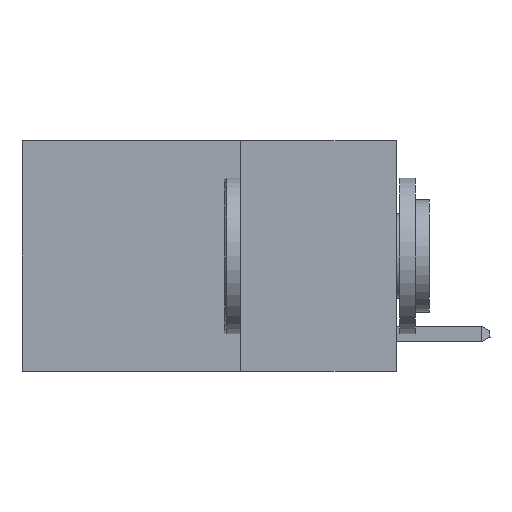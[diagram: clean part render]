
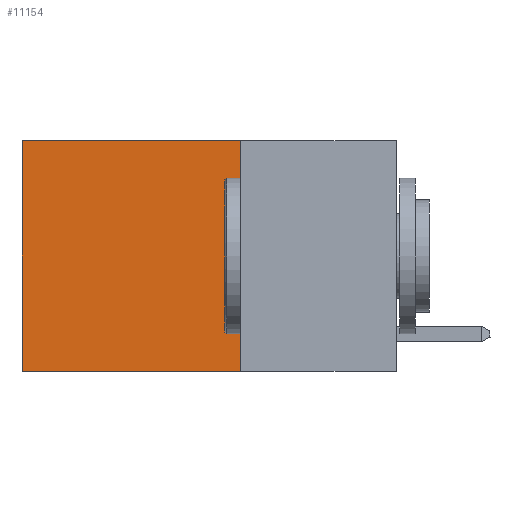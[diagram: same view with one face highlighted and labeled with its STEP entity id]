
A CAD part, left-side view. The second image highlights one B-rep face of the part: STEP entity #11154.
In plain terms, the highlighted planar face has unit normal (-1, 0, 0).
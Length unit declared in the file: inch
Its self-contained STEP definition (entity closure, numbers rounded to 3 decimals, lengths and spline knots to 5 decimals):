
#129 = ORIENTED_EDGE ( 'NONE', *, *, #913, .T. ) ;
#226 = ORIENTED_EDGE ( 'NONE', *, *, #10465, .F. ) ;
#417 = ORIENTED_EDGE ( 'NONE', *, *, #9781, .F. ) ;
#844 = ORIENTED_EDGE ( 'NONE', *, *, #8347, .T. ) ;
#913 = EDGE_CURVE ( 'NONE', #7312, #3012, #1045, .T. ) ;
#1045 = LINE ( 'NONE', #1157, #8351 ) ;
#1157 = CARTESIAN_POINT ( 'NONE',  ( 0.2625, 0.6, 0. ) ) ;
#1704 = DIRECTION ( 'NONE',  ( 1., 0., 0. ) ) ;
#1806 = DIRECTION ( 'NONE',  ( 0., 1., 0. ) ) ;
#2155 = VERTEX_POINT ( 'NONE', #4856 ) ;
#2411 = CARTESIAN_POINT ( 'NONE',  ( 0.2625, 0.6, 0. ) ) ;
#2602 = CARTESIAN_POINT ( 'NONE',  ( 0.2625, 0.25, 0. ) ) ;
#2667 = CARTESIAN_POINT ( 'NONE',  ( 0.2625, 0.25, -0.37 ) ) ;
#3012 = VERTEX_POINT ( 'NONE', #6896 ) ;
#3633 = VERTEX_POINT ( 'NONE', #2667 ) ;
#4054 = CARTESIAN_POINT ( 'NONE',  ( 0.2625, 0.25, 0. ) ) ;
#4080 = EDGE_LOOP ( 'NONE', ( #129, #226, #417, #844 ) ) ;
#4221 = LINE ( 'NONE', #9901, #6389 ) ;
#4833 = VECTOR ( 'NONE', #10342, 39.37008 ) ;
#4856 = CARTESIAN_POINT ( 'NONE',  ( 0.2625, 0.25, 0. ) ) ;
#6389 = VECTOR ( 'NONE', #1806, 39.37008 ) ;
#6429 = DIRECTION ( 'NONE',  ( 0., 0., -1. ) ) ;
#6542 = VECTOR ( 'NONE', #6429, 39.37008 ) ;
#6896 = CARTESIAN_POINT ( 'NONE',  ( 0.2625, 0.6, -0.37 ) ) ;
#7312 = VERTEX_POINT ( 'NONE', #2411 ) ;
#8087 = DIRECTION ( 'NONE',  ( 0., 0., -1. ) ) ;
#8347 = EDGE_CURVE ( 'NONE', #2155, #7312, #9624, .T. ) ;
#8351 = VECTOR ( 'NONE', #11444, 39.37008 ) ;
#9162 = FACE_OUTER_BOUND ( 'NONE', #4080, .T. ) ;
#9512 = AXIS2_PLACEMENT_3D ( 'NONE', #2602, #1704, #8087 ) ;
#9624 = LINE ( 'NONE', #4054, #4833 ) ;
#9781 = EDGE_CURVE ( 'NONE', #2155, #3633, #10945, .T. ) ;
#9901 = CARTESIAN_POINT ( 'NONE',  ( 0.2625, 0.25, -0.37 ) ) ;
#10342 = DIRECTION ( 'NONE',  ( 0., 1., 0. ) ) ;
#10465 = EDGE_CURVE ( 'NONE', #3633, #3012, #4221, .T. ) ;
#10687 = PLANE ( 'NONE',  #9512 ) ;
#10945 = LINE ( 'NONE', #11640, #6542 ) ;
#11154 = ADVANCED_FACE ( 'NONE', ( #9162 ), #10687, .F. ) ;
#11444 = DIRECTION ( 'NONE',  ( 0., 0., -1. ) ) ;
#11640 = CARTESIAN_POINT ( 'NONE',  ( 0.2625, 0.25, 0. ) ) ;
